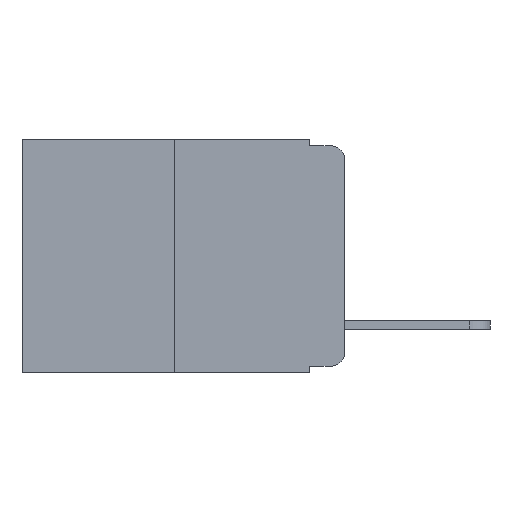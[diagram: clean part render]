
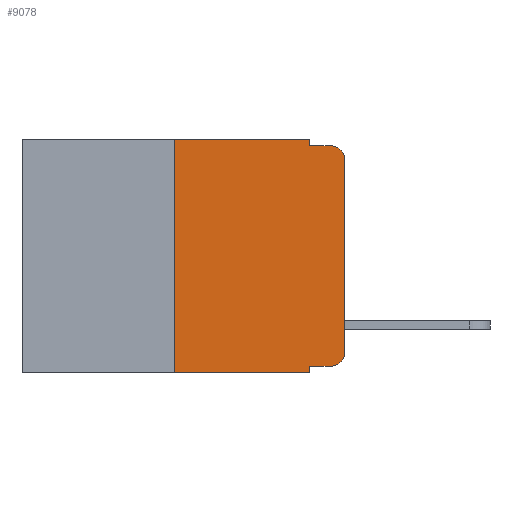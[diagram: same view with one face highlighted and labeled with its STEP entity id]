
A CAD part, left-side view. The second image highlights one B-rep face of the part: STEP entity #9078.
In plain terms, the highlighted planar face has unit normal (-1, 0, 0).
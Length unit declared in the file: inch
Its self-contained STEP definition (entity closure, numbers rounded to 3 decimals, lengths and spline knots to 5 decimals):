
#47 = DIRECTION ( 'NONE',  ( 0., 0., -1. ) ) ;
#403 = VECTOR ( 'NONE', #20712, 39.37008 ) ;
#508 = CARTESIAN_POINT ( 'NONE',  ( 0., 0.473, 0. ) ) ;
#561 = ORIENTED_EDGE ( 'NONE', *, *, #2173, .F. ) ;
#1248 = VECTOR ( 'NONE', #2436, 39.37008 ) ;
#1353 = ORIENTED_EDGE ( 'NONE', *, *, #2288, .T. ) ;
#1373 = CARTESIAN_POINT ( 'NONE',  ( 0., 0.02, -0.333 ) ) ;
#1527 = CARTESIAN_POINT ( 'NONE',  ( 0., 0.051, 0. ) ) ;
#1683 = VERTEX_POINT ( 'NONE', #13608 ) ;
#1827 = LINE ( 'NONE', #5692, #1248 ) ;
#2104 = EDGE_CURVE ( 'NONE', #10530, #19065, #11719, .T. ) ;
#2139 = EDGE_CURVE ( 'NONE', #6915, #10530, #14019, .T. ) ;
#2173 = EDGE_CURVE ( 'NONE', #6915, #20347, #8950, .T. ) ;
#2180 = EDGE_CURVE ( 'NONE', #1683, #21182, #17262, .T. ) ;
#2217 = EDGE_CURVE ( 'NONE', #15782, #8897, #21292, .T. ) ;
#2242 = DIRECTION ( 'NONE',  ( 0., -1., 0. ) ) ;
#2252 = EDGE_CURVE ( 'NONE', #8897, #4383, #1827, .T. ) ;
#2288 = EDGE_CURVE ( 'NONE', #4216, #4383, #18938, .T. ) ;
#2354 = CARTESIAN_POINT ( 'NONE',  ( 0., 0.473, -0.343 ) ) ;
#2372 = EDGE_CURVE ( 'NONE', #19065, #4216, #11699, .T. ) ;
#2436 = DIRECTION ( 'NONE',  ( 0., -1., 0. ) ) ;
#2678 = ORIENTED_EDGE ( 'NONE', *, *, #3232, .T. ) ;
#2799 = CARTESIAN_POINT ( 'NONE',  ( 0., 0., -0.313 ) ) ;
#3174 = ORIENTED_EDGE ( 'NONE', *, *, #11816, .F. ) ;
#3232 = EDGE_CURVE ( 'NONE', #1683, #20347, #20326, .T. ) ;
#3382 = CARTESIAN_POINT ( 'NONE',  ( 0., 0.051, -0.343 ) ) ;
#3492 = ORIENTED_EDGE ( 'NONE', *, *, #2139, .T. ) ;
#3498 = DIRECTION ( 'NONE',  ( 0., 0., 1. ) ) ;
#4216 = VERTEX_POINT ( 'NONE', #14747 ) ;
#4383 = VERTEX_POINT ( 'NONE', #12052 ) ;
#4519 = CARTESIAN_POINT ( 'NONE',  ( 0., 0.051, -0.333 ) ) ;
#4929 = DIRECTION ( 'NONE',  ( 0., 0., -1. ) ) ;
#4952 = DIRECTION ( 'NONE',  ( 1., 0., 0. ) ) ;
#4976 = ORIENTED_EDGE ( 'NONE', *, *, #2372, .T. ) ;
#5078 = PLANE ( 'NONE',  #20562 ) ;
#5618 = CARTESIAN_POINT ( 'NONE',  ( 0., 0.473, 0. ) ) ;
#5692 = CARTESIAN_POINT ( 'NONE',  ( 0., 0.051, -0.01 ) ) ;
#6433 = CARTESIAN_POINT ( 'NONE',  ( 0., 0.051, -0.333 ) ) ;
#6589 = EDGE_LOOP ( 'NONE', ( #4976, #1353, #15512, #9138, #3174, #16439, #2678, #561, #3492, #10756 ) ) ;
#6915 = VERTEX_POINT ( 'NONE', #6433 ) ;
#6971 = VECTOR ( 'NONE', #20513, 39.37008 ) ;
#7266 = VECTOR ( 'NONE', #20844, 39.37008 ) ;
#7757 = AXIS2_PLACEMENT_3D ( 'NONE', #8152, #15290, #15183 ) ;
#7903 = LINE ( 'NONE', #508, #16354 ) ;
#8152 = CARTESIAN_POINT ( 'NONE',  ( 0., 0.02, -0.03 ) ) ;
#8217 = AXIS2_PLACEMENT_3D ( 'NONE', #21217, #13377, #21193 ) ;
#8383 = VECTOR ( 'NONE', #3498, 39.37008 ) ;
#8897 = VERTEX_POINT ( 'NONE', #10898 ) ;
#8950 = LINE ( 'NONE', #20135, #17745 ) ;
#9078 = ADVANCED_FACE ( 'NONE', ( #11682 ), #5078, .F. ) ;
#9138 = ORIENTED_EDGE ( 'NONE', *, *, #2217, .F. ) ;
#10530 = VERTEX_POINT ( 'NONE', #1373 ) ;
#10756 = ORIENTED_EDGE ( 'NONE', *, *, #2104, .T. ) ;
#10898 = CARTESIAN_POINT ( 'NONE',  ( 0., 0.051, -0.01 ) ) ;
#11682 = FACE_OUTER_BOUND ( 'NONE', #6589, .T. ) ;
#11699 = LINE ( 'NONE', #20259, #6971 ) ;
#11719 = CIRCLE ( 'NONE', #8217, 0.02 ) ;
#11816 = EDGE_CURVE ( 'NONE', #21182, #15782, #7903, .T. ) ;
#12052 = CARTESIAN_POINT ( 'NONE',  ( 0., 0.02, -0.01 ) ) ;
#12679 = CARTESIAN_POINT ( 'NONE',  ( 0., 0.25, 0. ) ) ;
#13049 = DIRECTION ( 'NONE',  ( 0., -1., 0. ) ) ;
#13377 = DIRECTION ( 'NONE',  ( -1., 0., 0. ) ) ;
#13608 = CARTESIAN_POINT ( 'NONE',  ( 0., 0.25, -0.343 ) ) ;
#14019 = LINE ( 'NONE', #4519, #403 ) ;
#14747 = CARTESIAN_POINT ( 'NONE',  ( 0., 0., -0.03 ) ) ;
#15183 = DIRECTION ( 'NONE',  ( 0., 0., -1. ) ) ;
#15290 = DIRECTION ( 'NONE',  ( -1., 0., 0. ) ) ;
#15512 = ORIENTED_EDGE ( 'NONE', *, *, #2252, .F. ) ;
#15710 = VECTOR ( 'NONE', #2242, 39.37008 ) ;
#15782 = VERTEX_POINT ( 'NONE', #1527 ) ;
#16354 = VECTOR ( 'NONE', #13049, 39.37008 ) ;
#16439 = ORIENTED_EDGE ( 'NONE', *, *, #2180, .F. ) ;
#16857 = CARTESIAN_POINT ( 'NONE',  ( 0., 0.25, 0. ) ) ;
#17262 = LINE ( 'NONE', #12679, #8383 ) ;
#17745 = VECTOR ( 'NONE', #47, 39.37008 ) ;
#18938 = CIRCLE ( 'NONE', #7757, 0.02 ) ;
#19065 = VERTEX_POINT ( 'NONE', #2799 ) ;
#20135 = CARTESIAN_POINT ( 'NONE',  ( 0., 0.051, 0. ) ) ;
#20259 = CARTESIAN_POINT ( 'NONE',  ( 0., 0., 0. ) ) ;
#20287 = CARTESIAN_POINT ( 'NONE',  ( 0., 0.051, 0. ) ) ;
#20326 = LINE ( 'NONE', #2354, #15710 ) ;
#20347 = VERTEX_POINT ( 'NONE', #3382 ) ;
#20513 = DIRECTION ( 'NONE',  ( 0., 0., 1. ) ) ;
#20562 = AXIS2_PLACEMENT_3D ( 'NONE', #5618, #4952, #4929 ) ;
#20712 = DIRECTION ( 'NONE',  ( 0., -1., 0. ) ) ;
#20844 = DIRECTION ( 'NONE',  ( 0., 0., -1. ) ) ;
#21182 = VERTEX_POINT ( 'NONE', #16857 ) ;
#21193 = DIRECTION ( 'NONE',  ( 0., 0., -1. ) ) ;
#21217 = CARTESIAN_POINT ( 'NONE',  ( 0., 0.02, -0.313 ) ) ;
#21292 = LINE ( 'NONE', #20287, #7266 ) ;
